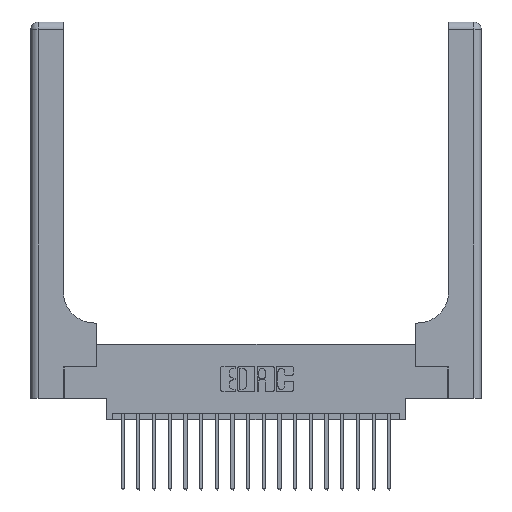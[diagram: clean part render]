
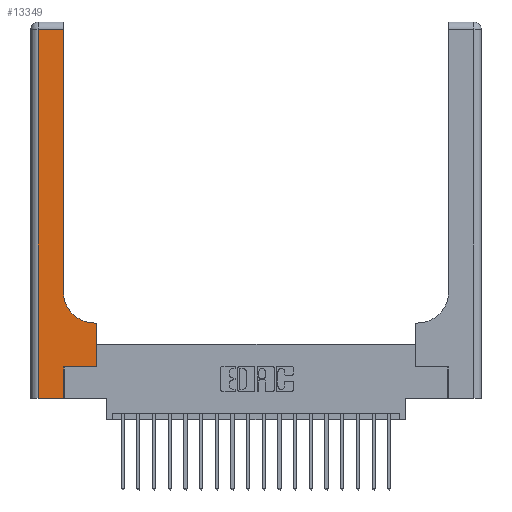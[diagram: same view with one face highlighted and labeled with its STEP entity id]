
A CAD part, top view. The second image highlights one B-rep face of the part: STEP entity #13349.
In plain terms, the highlighted planar face has unit normal (0, 0, 1).
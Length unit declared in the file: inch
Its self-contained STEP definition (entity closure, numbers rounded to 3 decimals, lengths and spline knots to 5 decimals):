
#348 = ORIENTED_EDGE ( 'NONE', *, *, #9551, .T. ) ;
#480 = VERTEX_POINT ( 'NONE', #607 ) ;
#607 = CARTESIAN_POINT ( 'NONE',  ( 0.51, 0.6, 0.37 ) ) ;
#963 = CARTESIAN_POINT ( 'NONE',  ( 0., 0., 0.37 ) ) ;
#1257 = CIRCLE ( 'NONE', #15989, 0.25 ) ;
#1507 = VECTOR ( 'NONE', #5144, 39.37008 ) ;
#1947 = LINE ( 'NONE', #11899, #4561 ) ;
#2148 = DIRECTION ( 'NONE',  ( 0., -1., 0. ) ) ;
#2178 = LINE ( 'NONE', #9927, #1507 ) ;
#2462 = DIRECTION ( 'NONE',  ( 0., 1., 0. ) ) ;
#2568 = CARTESIAN_POINT ( 'NONE',  ( 0.528, 0.25, 0.37 ) ) ;
#2748 = DIRECTION ( 'NONE',  ( 1., 0., 0. ) ) ;
#3482 = CARTESIAN_POINT ( 'NONE',  ( 0.26, 0.85, 0.37 ) ) ;
#4359 = VECTOR ( 'NONE', #14846, 39.37008 ) ;
#4409 = CARTESIAN_POINT ( 'NONE',  ( 0.265, 0., 0.37 ) ) ;
#4561 = VECTOR ( 'NONE', #2148, 39.37008 ) ;
#5144 = DIRECTION ( 'NONE',  ( 0., 1., 0. ) ) ;
#5495 = VECTOR ( 'NONE', #2748, 39.37008 ) ;
#5682 = ORIENTED_EDGE ( 'NONE', *, *, #6779, .T. ) ;
#6231 = ORIENTED_EDGE ( 'NONE', *, *, #6941, .T. ) ;
#6530 = VERTEX_POINT ( 'NONE', #8874 ) ;
#6757 = CARTESIAN_POINT ( 'NONE',  ( 0.528, 0.6, 0.37 ) ) ;
#6779 = EDGE_CURVE ( 'NONE', #15891, #13440, #1947, .T. ) ;
#6915 = PLANE ( 'NONE',  #7260 ) ;
#6941 = EDGE_CURVE ( 'NONE', #14141, #8342, #18640, .T. ) ;
#7260 = AXIS2_PLACEMENT_3D ( 'NONE', #16475, #13306, #19727 ) ;
#7453 = DIRECTION ( 'NONE',  ( -1., 0., 0. ) ) ;
#8156 = ORIENTED_EDGE ( 'NONE', *, *, #9981, .T. ) ;
#8173 = CARTESIAN_POINT ( 'NONE',  ( 0.51, 0.85, 0.37 ) ) ;
#8240 = VERTEX_POINT ( 'NONE', #4409 ) ;
#8342 = VERTEX_POINT ( 'NONE', #6757 ) ;
#8874 = CARTESIAN_POINT ( 'NONE',  ( 0.26, 2.94, 0.37 ) ) ;
#9102 = EDGE_CURVE ( 'NONE', #20522, #6530, #2178, .T. ) ;
#9128 = LINE ( 'NONE', #18802, #11340 ) ;
#9320 = EDGE_CURVE ( 'NONE', #8240, #19527, #11932, .T. ) ;
#9551 = EDGE_CURVE ( 'NONE', #19527, #14141, #19382, .T. ) ;
#9804 = CARTESIAN_POINT ( 'NONE',  ( 0.265, 0.25, 0.37 ) ) ;
#9927 = CARTESIAN_POINT ( 'NONE',  ( 0.26, 3., 0.37 ) ) ;
#9981 = EDGE_CURVE ( 'NONE', #13440, #8240, #17114, .T. ) ;
#10045 = FACE_OUTER_BOUND ( 'NONE', #17210, .T. ) ;
#10234 = DIRECTION ( 'NONE',  ( 0., 1., 0. ) ) ;
#10627 = EDGE_CURVE ( 'NONE', #6530, #15891, #9128, .T. ) ;
#10875 = CARTESIAN_POINT ( 'NONE',  ( 0.06, 2.94, 0.37 ) ) ;
#10950 = DIRECTION ( 'NONE',  ( -1., 0., 0. ) ) ;
#11062 = CARTESIAN_POINT ( 'NONE',  ( 0.265, 0.25, 0.37 ) ) ;
#11064 = LINE ( 'NONE', #17900, #19708 ) ;
#11324 = ORIENTED_EDGE ( 'NONE', *, *, #13158, .T. ) ;
#11340 = VECTOR ( 'NONE', #7453, 39.37008 ) ;
#11899 = CARTESIAN_POINT ( 'NONE',  ( 0.06, 3., 0.37 ) ) ;
#11932 = LINE ( 'NONE', #13709, #15285 ) ;
#12801 = DIRECTION ( 'NONE',  ( 0., 0., -1. ) ) ;
#13158 = EDGE_CURVE ( 'NONE', #480, #20522, #1257, .T. ) ;
#13306 = DIRECTION ( 'NONE',  ( 0., 0., -1. ) ) ;
#13349 = ADVANCED_FACE ( 'NONE', ( #10045 ), #6915, .F. ) ;
#13440 = VERTEX_POINT ( 'NONE', #20042 ) ;
#13642 = CARTESIAN_POINT ( 'NONE',  ( 0.528, 0.25, 0.37 ) ) ;
#13709 = CARTESIAN_POINT ( 'NONE',  ( 0.265, 0., 0.37 ) ) ;
#14015 = EDGE_CURVE ( 'NONE', #8342, #480, #11064, .T. ) ;
#14127 = ORIENTED_EDGE ( 'NONE', *, *, #9320, .T. ) ;
#14141 = VERTEX_POINT ( 'NONE', #13642 ) ;
#14846 = DIRECTION ( 'NONE',  ( 1., 0., 0. ) ) ;
#15285 = VECTOR ( 'NONE', #10234, 39.37008 ) ;
#15891 = VERTEX_POINT ( 'NONE', #10875 ) ;
#15926 = VECTOR ( 'NONE', #2462, 39.37008 ) ;
#15989 = AXIS2_PLACEMENT_3D ( 'NONE', #8173, #12801, #19222 ) ;
#16475 = CARTESIAN_POINT ( 'NONE',  ( 0., 3., 0.37 ) ) ;
#17114 = LINE ( 'NONE', #963, #5495 ) ;
#17207 = ORIENTED_EDGE ( 'NONE', *, *, #9102, .T. ) ;
#17210 = EDGE_LOOP ( 'NONE', ( #17207, #19245, #5682, #8156, #14127, #348, #6231, #18086, #11324 ) ) ;
#17900 = CARTESIAN_POINT ( 'NONE',  ( 0.26, 0.6, 0.37 ) ) ;
#18086 = ORIENTED_EDGE ( 'NONE', *, *, #14015, .T. ) ;
#18640 = LINE ( 'NONE', #2568, #15926 ) ;
#18802 = CARTESIAN_POINT ( 'NONE',  ( 0., 2.94, 0.37 ) ) ;
#19222 = DIRECTION ( 'NONE',  ( 1., 0., 0. ) ) ;
#19245 = ORIENTED_EDGE ( 'NONE', *, *, #10627, .T. ) ;
#19382 = LINE ( 'NONE', #9804, #4359 ) ;
#19527 = VERTEX_POINT ( 'NONE', #11062 ) ;
#19708 = VECTOR ( 'NONE', #10950, 39.37008 ) ;
#19727 = DIRECTION ( 'NONE',  ( -1., 0., 0. ) ) ;
#20042 = CARTESIAN_POINT ( 'NONE',  ( 0.06, 0., 0.37 ) ) ;
#20522 = VERTEX_POINT ( 'NONE', #3482 ) ;
